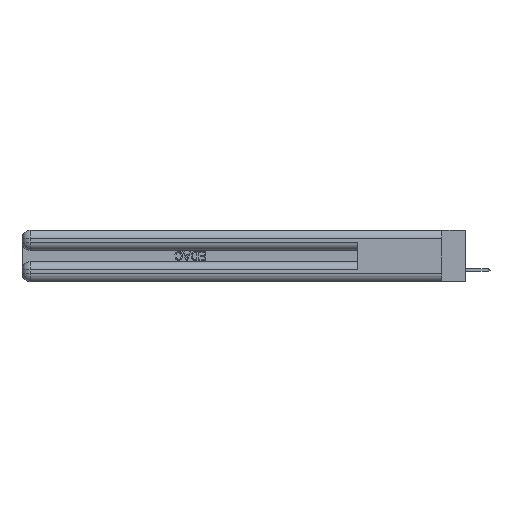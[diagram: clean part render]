
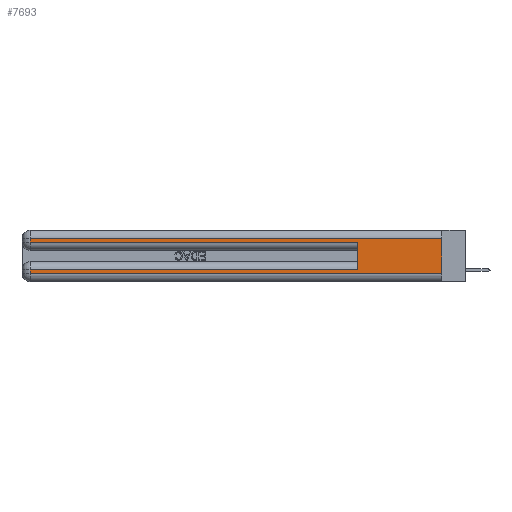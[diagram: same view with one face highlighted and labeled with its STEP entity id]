
A CAD part, left-side view. The second image highlights one B-rep face of the part: STEP entity #7693.
In plain terms, the highlighted planar face has unit normal (-1, 0, 0).
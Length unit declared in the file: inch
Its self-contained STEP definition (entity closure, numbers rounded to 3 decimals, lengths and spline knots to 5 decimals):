
#426 = VECTOR ( 'NONE', #35343, 39.37008 ) ;
#1207 = DIRECTION ( 'NONE',  ( 0., 0., -1. ) ) ;
#4086 = ORIENTED_EDGE ( 'NONE', *, *, #18510, .T. ) ;
#4247 = VERTEX_POINT ( 'NONE', #13200 ) ;
#4376 = VERTEX_POINT ( 'NONE', #16596 ) ;
#4805 = CARTESIAN_POINT ( 'NONE',  ( 0., 2.94, 0.085 ) ) ;
#5619 = ORIENTED_EDGE ( 'NONE', *, *, #6511, .T. ) ;
#6356 = CARTESIAN_POINT ( 'NONE',  ( 0., 0.6, 0.145 ) ) ;
#6511 = EDGE_CURVE ( 'NONE', #18325, #23344, #23792, .T. ) ;
#6939 = CARTESIAN_POINT ( 'NONE',  ( 0., 2.94, 0.37 ) ) ;
#7693 = ADVANCED_FACE ( 'NONE', ( #18386 ), #23781, .F. ) ;
#8398 = ORIENTED_EDGE ( 'NONE', *, *, #19325, .T. ) ;
#8988 = CARTESIAN_POINT ( 'NONE',  ( 0., 0.6, 0.085 ) ) ;
#9859 = LINE ( 'NONE', #6939, #29771 ) ;
#10478 = DIRECTION ( 'NONE',  ( 0., 0., -1. ) ) ;
#10560 = DIRECTION ( 'NONE',  ( 0., 0., -1. ) ) ;
#10751 = CARTESIAN_POINT ( 'NONE',  ( 0., 0., 0.37 ) ) ;
#12425 = DIRECTION ( 'NONE',  ( 0., 1., 0. ) ) ;
#12727 = CARTESIAN_POINT ( 'NONE',  ( 0., 0., 0.085 ) ) ;
#13200 = CARTESIAN_POINT ( 'NONE',  ( 0., 0.6, 0.285 ) ) ;
#14747 = AXIS2_PLACEMENT_3D ( 'NONE', #30711, #19707, #40573 ) ;
#14761 = EDGE_CURVE ( 'NONE', #15206, #4247, #32107, .T. ) ;
#15206 = VERTEX_POINT ( 'NONE', #8988 ) ;
#15646 = VERTEX_POINT ( 'NONE', #4805 ) ;
#16151 = CARTESIAN_POINT ( 'NONE',  ( 0., 0., 0.06 ) ) ;
#16596 = CARTESIAN_POINT ( 'NONE',  ( 0., 2.94, 0.285 ) ) ;
#17087 = VECTOR ( 'NONE', #23009, 39.37008 ) ;
#17725 = ORIENTED_EDGE ( 'NONE', *, *, #22899, .F. ) ;
#18325 = VERTEX_POINT ( 'NONE', #35602 ) ;
#18386 = FACE_OUTER_BOUND ( 'NONE', #32253, .T. ) ;
#18510 = EDGE_CURVE ( 'NONE', #4376, #4247, #34519, .T. ) ;
#19042 = VECTOR ( 'NONE', #12425, 39.37008 ) ;
#19325 = EDGE_CURVE ( 'NONE', #24857, #4376, #38370, .T. ) ;
#19707 = DIRECTION ( 'NONE',  ( 1., 0., 0. ) ) ;
#21327 = DIRECTION ( 'NONE',  ( 0., -1., 0. ) ) ;
#21382 = LINE ( 'NONE', #34920, #426 ) ;
#22790 = ORIENTED_EDGE ( 'NONE', *, *, #14761, .F. ) ;
#22899 = EDGE_CURVE ( 'NONE', #35859, #23344, #25129, .T. ) ;
#23009 = DIRECTION ( 'NONE',  ( 0., 0., 1. ) ) ;
#23344 = VERTEX_POINT ( 'NONE', #16151 ) ;
#23781 = PLANE ( 'NONE',  #14747 ) ;
#23792 = LINE ( 'NONE', #38445, #24302 ) ;
#24302 = VECTOR ( 'NONE', #21327, 39.37008 ) ;
#24857 = VERTEX_POINT ( 'NONE', #35963 ) ;
#25129 = LINE ( 'NONE', #10751, #35873 ) ;
#27143 = VECTOR ( 'NONE', #1207, 39.37008 ) ;
#29771 = VECTOR ( 'NONE', #10560, 39.37008 ) ;
#30204 = VECTOR ( 'NONE', #40037, 39.37008 ) ;
#30711 = CARTESIAN_POINT ( 'NONE',  ( 0., 0., 0.37 ) ) ;
#31285 = CARTESIAN_POINT ( 'NONE',  ( 0., 2.94, 0.37 ) ) ;
#31910 = ORIENTED_EDGE ( 'NONE', *, *, #34383, .T. ) ;
#32107 = LINE ( 'NONE', #6356, #17087 ) ;
#32253 = EDGE_LOOP ( 'NONE', ( #17725, #33235, #8398, #4086, #22790, #41894, #31910, #5619 ) ) ;
#33031 = CARTESIAN_POINT ( 'NONE',  ( 0., 0., 0.285 ) ) ;
#33235 = ORIENTED_EDGE ( 'NONE', *, *, #41064, .T. ) ;
#34383 = EDGE_CURVE ( 'NONE', #15646, #18325, #9859, .T. ) ;
#34519 = LINE ( 'NONE', #33031, #30204 ) ;
#34920 = CARTESIAN_POINT ( 'NONE',  ( 0., 0., 0.31 ) ) ;
#35343 = DIRECTION ( 'NONE',  ( 0., 1., 0. ) ) ;
#35602 = CARTESIAN_POINT ( 'NONE',  ( 0., 2.94, 0.06 ) ) ;
#35859 = VERTEX_POINT ( 'NONE', #39433 ) ;
#35873 = VECTOR ( 'NONE', #10478, 39.37008 ) ;
#35963 = CARTESIAN_POINT ( 'NONE',  ( 0., 2.94, 0.31 ) ) ;
#37859 = LINE ( 'NONE', #12727, #19042 ) ;
#38370 = LINE ( 'NONE', #31285, #27143 ) ;
#38445 = CARTESIAN_POINT ( 'NONE',  ( 0., 0., 0.06 ) ) ;
#39433 = CARTESIAN_POINT ( 'NONE',  ( 0., 0., 0.31 ) ) ;
#40037 = DIRECTION ( 'NONE',  ( 0., -1., 0. ) ) ;
#40573 = DIRECTION ( 'NONE',  ( 0., 0., -1. ) ) ;
#41064 = EDGE_CURVE ( 'NONE', #35859, #24857, #21382, .T. ) ;
#41894 = ORIENTED_EDGE ( 'NONE', *, *, #43773, .T. ) ;
#43773 = EDGE_CURVE ( 'NONE', #15206, #15646, #37859, .T. ) ;
